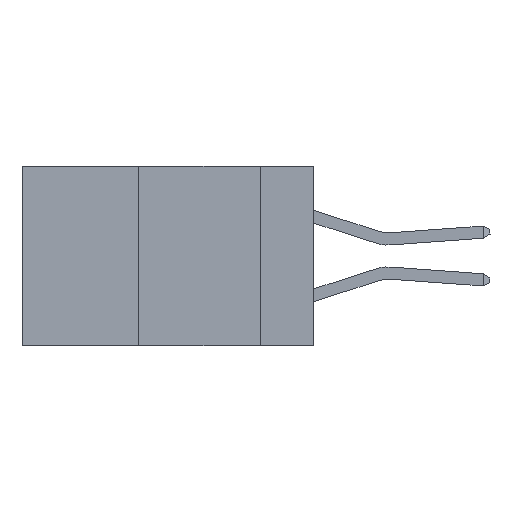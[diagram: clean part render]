
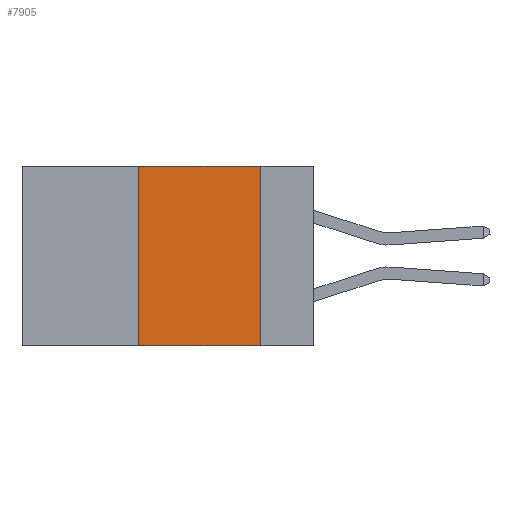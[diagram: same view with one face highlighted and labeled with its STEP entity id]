
A CAD part, left-side view. The second image highlights one B-rep face of the part: STEP entity #7905.
In plain terms, the highlighted planar face has unit normal (-1, 0, 0).
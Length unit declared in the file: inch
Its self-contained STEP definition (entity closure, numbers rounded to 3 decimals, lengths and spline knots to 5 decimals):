
#107 = VECTOR ( 'NONE', #387, 39.37008 ) ;
#252 = VECTOR ( 'NONE', #9186, 39.37008 ) ;
#387 = DIRECTION ( 'NONE',  ( 0., 0., -1. ) ) ;
#584 = DIRECTION ( 'NONE',  ( 0., 0., -1. ) ) ;
#785 = FACE_OUTER_BOUND ( 'NONE', #7463, .T. ) ;
#991 = VECTOR ( 'NONE', #2987, 39.37008 ) ;
#1204 = CARTESIAN_POINT ( 'NONE',  ( 0., 0.11, 0. ) ) ;
#1847 = EDGE_CURVE ( 'NONE', #7934, #5679, #8355, .T. ) ;
#2216 = ORIENTED_EDGE ( 'NONE', *, *, #1847, .T. ) ;
#2239 = PLANE ( 'NONE',  #9206 ) ;
#2411 = VERTEX_POINT ( 'NONE', #9939 ) ;
#2763 = CARTESIAN_POINT ( 'NONE',  ( 0., 0.11, 0. ) ) ;
#2945 = CARTESIAN_POINT ( 'NONE',  ( 0., 0.6, -0.37 ) ) ;
#2987 = DIRECTION ( 'NONE',  ( 0., 0., 1. ) ) ;
#3037 = LINE ( 'NONE', #8701, #991 ) ;
#3091 = DIRECTION ( 'NONE',  ( 0., -1., 0. ) ) ;
#3152 = EDGE_CURVE ( 'NONE', #2411, #3285, #6752, .T. ) ;
#3285 = VERTEX_POINT ( 'NONE', #1204 ) ;
#3632 = ORIENTED_EDGE ( 'NONE', *, *, #6975, .F. ) ;
#4007 = ORIENTED_EDGE ( 'NONE', *, *, #3152, .F. ) ;
#4040 = EDGE_CURVE ( 'NONE', #3285, #5679, #4307, .T. ) ;
#4200 = VECTOR ( 'NONE', #3091, 39.37008 ) ;
#4307 = LINE ( 'NONE', #2763, #107 ) ;
#5251 = CARTESIAN_POINT ( 'NONE',  ( 0., 0.11, -0.37 ) ) ;
#5274 = CARTESIAN_POINT ( 'NONE',  ( 0., 0.6, 0. ) ) ;
#5679 = VERTEX_POINT ( 'NONE', #5251 ) ;
#6752 = LINE ( 'NONE', #5274, #252 ) ;
#6975 = EDGE_CURVE ( 'NONE', #7934, #2411, #3037, .T. ) ;
#7463 = EDGE_LOOP ( 'NONE', ( #7484, #4007, #3632, #2216 ) ) ;
#7484 = ORIENTED_EDGE ( 'NONE', *, *, #4040, .F. ) ;
#7706 = DIRECTION ( 'NONE',  ( 1., 0., 0. ) ) ;
#7865 = CARTESIAN_POINT ( 'NONE',  ( 0., 0.6, 0. ) ) ;
#7905 = ADVANCED_FACE ( 'NONE', ( #785 ), #2239, .F. ) ;
#7934 = VERTEX_POINT ( 'NONE', #9190 ) ;
#8355 = LINE ( 'NONE', #2945, #4200 ) ;
#8701 = CARTESIAN_POINT ( 'NONE',  ( 0., 0.36, 0. ) ) ;
#9186 = DIRECTION ( 'NONE',  ( 0., -1., 0. ) ) ;
#9190 = CARTESIAN_POINT ( 'NONE',  ( 0., 0.36, -0.37 ) ) ;
#9206 = AXIS2_PLACEMENT_3D ( 'NONE', #7865, #7706, #584 ) ;
#9939 = CARTESIAN_POINT ( 'NONE',  ( 0., 0.36, 0. ) ) ;
